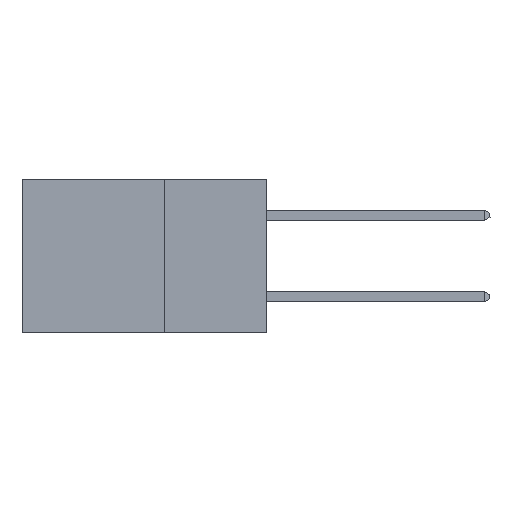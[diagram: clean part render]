
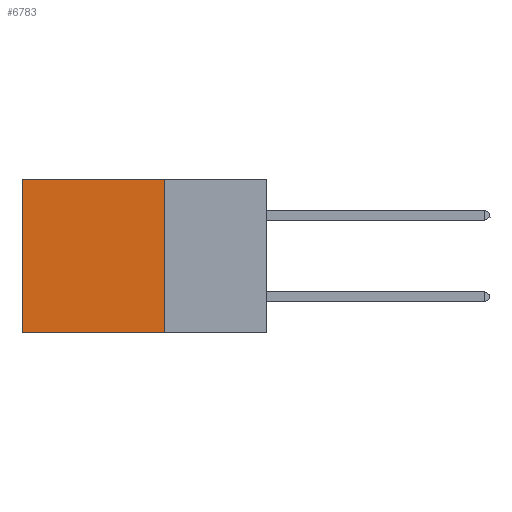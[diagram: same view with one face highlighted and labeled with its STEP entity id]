
A CAD part, left-side view. The second image highlights one B-rep face of the part: STEP entity #6783.
In plain terms, the highlighted planar face has unit normal (-1, 0, 0).
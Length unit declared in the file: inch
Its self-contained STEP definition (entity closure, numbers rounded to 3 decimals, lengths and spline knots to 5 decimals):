
#149 = CARTESIAN_POINT ( 'NONE',  ( 0.2875, 0.25, 0. ) ) ;
#392 = DIRECTION ( 'NONE',  ( 0., 0., -1. ) ) ;
#468 = VECTOR ( 'NONE', #1519, 39.37008 ) ;
#813 = VERTEX_POINT ( 'NONE', #7544 ) ;
#938 = VERTEX_POINT ( 'NONE', #5616 ) ;
#1519 = DIRECTION ( 'NONE',  ( 0., 1., 0. ) ) ;
#1538 = EDGE_CURVE ( 'NONE', #8468, #5584, #4110, .T. ) ;
#1808 = LINE ( 'NONE', #149, #468 ) ;
#1809 = CARTESIAN_POINT ( 'NONE',  ( 0.2875, 0.25, -0.375 ) ) ;
#1853 = EDGE_LOOP ( 'NONE', ( #5188, #2778, #3790, #4027 ) ) ;
#2728 = EDGE_CURVE ( 'NONE', #813, #938, #7396, .T. ) ;
#2778 = ORIENTED_EDGE ( 'NONE', *, *, #7916, .F. ) ;
#3024 = FACE_OUTER_BOUND ( 'NONE', #1853, .T. ) ;
#3267 = CARTESIAN_POINT ( 'NONE',  ( 0.2875, 0.25, -0.375 ) ) ;
#3706 = CARTESIAN_POINT ( 'NONE',  ( 0.2875, 0.25, -0.375 ) ) ;
#3790 = ORIENTED_EDGE ( 'NONE', *, *, #1538, .F. ) ;
#4027 = ORIENTED_EDGE ( 'NONE', *, *, #4936, .T. ) ;
#4110 = LINE ( 'NONE', #3267, #5659 ) ;
#4821 = CARTESIAN_POINT ( 'NONE',  ( 0.2875, 0.25, 0. ) ) ;
#4936 = EDGE_CURVE ( 'NONE', #8468, #813, #1808, .T. ) ;
#5051 = DIRECTION ( 'NONE',  ( 1., 0., 0. ) ) ;
#5188 = ORIENTED_EDGE ( 'NONE', *, *, #2728, .T. ) ;
#5399 = VECTOR ( 'NONE', #5522, 39.37008 ) ;
#5522 = DIRECTION ( 'NONE',  ( 0., 1., 0. ) ) ;
#5584 = VERTEX_POINT ( 'NONE', #3706 ) ;
#5616 = CARTESIAN_POINT ( 'NONE',  ( 0.2875, 0.6, -0.375 ) ) ;
#5639 = VECTOR ( 'NONE', #7830, 39.37008 ) ;
#5659 = VECTOR ( 'NONE', #5967, 39.37008 ) ;
#5967 = DIRECTION ( 'NONE',  ( 0., 0., -1. ) ) ;
#6396 = CARTESIAN_POINT ( 'NONE',  ( 0.2875, 0.6, -0.375 ) ) ;
#6783 = ADVANCED_FACE ( 'NONE', ( #3024 ), #7095, .F. ) ;
#7095 = PLANE ( 'NONE',  #7714 ) ;
#7163 = LINE ( 'NONE', #8166, #5399 ) ;
#7396 = LINE ( 'NONE', #6396, #5639 ) ;
#7544 = CARTESIAN_POINT ( 'NONE',  ( 0.2875, 0.6, 0. ) ) ;
#7714 = AXIS2_PLACEMENT_3D ( 'NONE', #1809, #5051, #392 ) ;
#7830 = DIRECTION ( 'NONE',  ( 0., 0., -1. ) ) ;
#7916 = EDGE_CURVE ( 'NONE', #5584, #938, #7163, .T. ) ;
#8166 = CARTESIAN_POINT ( 'NONE',  ( 0.2875, 0.25, -0.375 ) ) ;
#8468 = VERTEX_POINT ( 'NONE', #4821 ) ;
